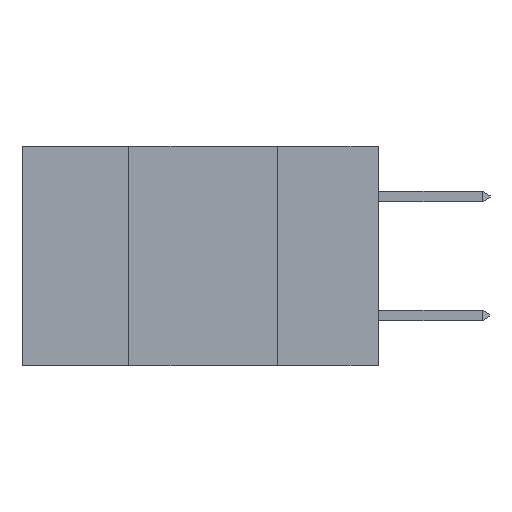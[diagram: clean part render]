
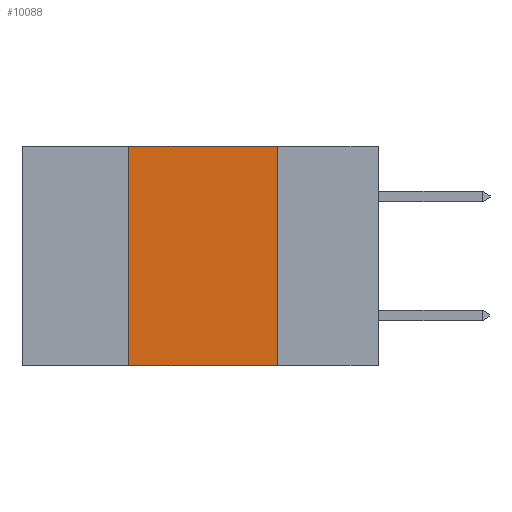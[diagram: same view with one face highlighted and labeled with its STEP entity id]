
A CAD part, left-side view. The second image highlights one B-rep face of the part: STEP entity #10088.
In plain terms, the highlighted planar face has unit normal (-1, 0, 0).
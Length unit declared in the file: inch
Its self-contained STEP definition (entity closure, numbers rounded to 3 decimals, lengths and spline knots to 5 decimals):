
#1688 = VECTOR ( 'NONE', #10511, 39.37008 ) ;
#1744 = VERTEX_POINT ( 'NONE', #8515 ) ;
#1795 = EDGE_CURVE ( 'NONE', #1744, #3295, #11676, .T. ) ;
#1812 = PLANE ( 'NONE',  #4726 ) ;
#2137 = EDGE_CURVE ( 'NONE', #8190, #1744, #3091, .T. ) ;
#2715 = DIRECTION ( 'NONE',  ( 0., 0., -1. ) ) ;
#2901 = EDGE_LOOP ( 'NONE', ( #8429, #6500, #6219, #6080 ) ) ;
#3091 = LINE ( 'NONE', #8601, #7906 ) ;
#3295 = VERTEX_POINT ( 'NONE', #10895 ) ;
#3565 = CARTESIAN_POINT ( 'NONE',  ( 0., 0.42, -0.37 ) ) ;
#3660 = VECTOR ( 'NONE', #11528, 39.37008 ) ;
#4240 = DIRECTION ( 'NONE',  ( 0., -1., 0. ) ) ;
#4726 = AXIS2_PLACEMENT_3D ( 'NONE', #8432, #8478, #2715 ) ;
#5139 = VERTEX_POINT ( 'NONE', #3565 ) ;
#5811 = CARTESIAN_POINT ( 'NONE',  ( 0., 0.42, 0. ) ) ;
#5925 = FACE_OUTER_BOUND ( 'NONE', #2901, .T. ) ;
#6080 = ORIENTED_EDGE ( 'NONE', *, *, #9131, .T. ) ;
#6219 = ORIENTED_EDGE ( 'NONE', *, *, #8329, .F. ) ;
#6277 = LINE ( 'NONE', #5811, #3660 ) ;
#6500 = ORIENTED_EDGE ( 'NONE', *, *, #2137, .F. ) ;
#7132 = VECTOR ( 'NONE', #9890, 39.37008 ) ;
#7906 = VECTOR ( 'NONE', #4240, 39.37008 ) ;
#8190 = VERTEX_POINT ( 'NONE', #9802 ) ;
#8319 = CARTESIAN_POINT ( 'NONE',  ( 0., 0.17, 0. ) ) ;
#8329 = EDGE_CURVE ( 'NONE', #5139, #8190, #6277, .T. ) ;
#8429 = ORIENTED_EDGE ( 'NONE', *, *, #1795, .F. ) ;
#8432 = CARTESIAN_POINT ( 'NONE',  ( 0., 0.6, 0. ) ) ;
#8478 = DIRECTION ( 'NONE',  ( 1., 0., 0. ) ) ;
#8515 = CARTESIAN_POINT ( 'NONE',  ( 0., 0.17, 0. ) ) ;
#8601 = CARTESIAN_POINT ( 'NONE',  ( 0., 0.6, 0. ) ) ;
#9131 = EDGE_CURVE ( 'NONE', #5139, #3295, #12034, .T. ) ;
#9802 = CARTESIAN_POINT ( 'NONE',  ( 0., 0.42, 0. ) ) ;
#9890 = DIRECTION ( 'NONE',  ( 0., -1., 0. ) ) ;
#10088 = ADVANCED_FACE ( 'NONE', ( #5925 ), #1812, .F. ) ;
#10511 = DIRECTION ( 'NONE',  ( 0., 0., -1. ) ) ;
#10779 = CARTESIAN_POINT ( 'NONE',  ( 0., 0.6, -0.37 ) ) ;
#10895 = CARTESIAN_POINT ( 'NONE',  ( 0., 0.17, -0.37 ) ) ;
#11528 = DIRECTION ( 'NONE',  ( 0., 0., 1. ) ) ;
#11676 = LINE ( 'NONE', #8319, #1688 ) ;
#12034 = LINE ( 'NONE', #10779, #7132 ) ;
